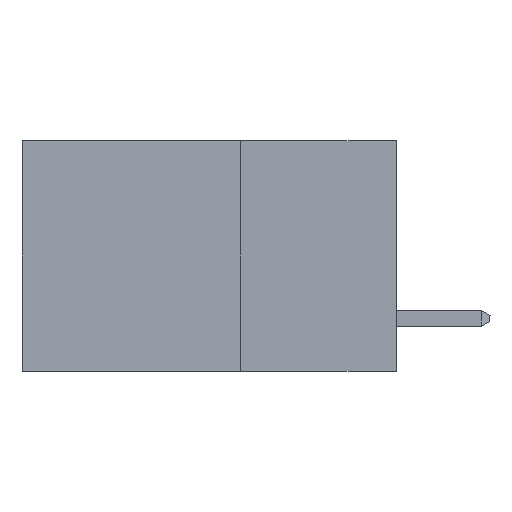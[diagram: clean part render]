
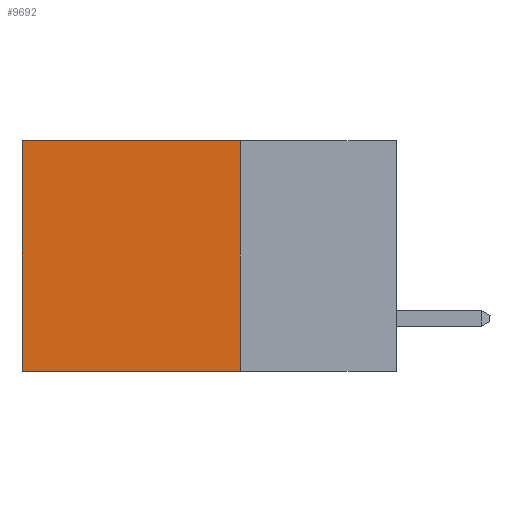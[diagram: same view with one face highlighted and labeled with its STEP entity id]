
A CAD part, left-side view. The second image highlights one B-rep face of the part: STEP entity #9692.
In plain terms, the highlighted planar face has unit normal (-1, 0, 0).
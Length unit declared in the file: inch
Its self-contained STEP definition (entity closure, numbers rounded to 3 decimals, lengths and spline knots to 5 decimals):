
#252 = VECTOR ( 'NONE', #7902, 39.37008 ) ;
#567 = EDGE_LOOP ( 'NONE', ( #10667, #6656, #911, #1092 ) ) ;
#683 = CARTESIAN_POINT ( 'NONE',  ( 0.298, 0.6, -0.37 ) ) ;
#911 = ORIENTED_EDGE ( 'NONE', *, *, #4705, .F. ) ;
#1075 = VERTEX_POINT ( 'NONE', #6024 ) ;
#1092 = ORIENTED_EDGE ( 'NONE', *, *, #1733, .T. ) ;
#1318 = CARTESIAN_POINT ( 'NONE',  ( 0.298, 0.25, -0.37 ) ) ;
#1333 = CARTESIAN_POINT ( 'NONE',  ( 0.298, 0.25, 0. ) ) ;
#1408 = LINE ( 'NONE', #6724, #8051 ) ;
#1498 = FACE_OUTER_BOUND ( 'NONE', #567, .T. ) ;
#1511 = VERTEX_POINT ( 'NONE', #3135 ) ;
#1540 = CARTESIAN_POINT ( 'NONE',  ( 0.298, 0.25, 0. ) ) ;
#1733 = EDGE_CURVE ( 'NONE', #1075, #1511, #1964, .T. ) ;
#1777 = DIRECTION ( 'NONE',  ( 0., 0., -1. ) ) ;
#1964 = LINE ( 'NONE', #1540, #252 ) ;
#2083 = DIRECTION ( 'NONE',  ( 0., 1., 0. ) ) ;
#2366 = DIRECTION ( 'NONE',  ( 0., 0., -1. ) ) ;
#2425 = VERTEX_POINT ( 'NONE', #683 ) ;
#3135 = CARTESIAN_POINT ( 'NONE',  ( 0.298, 0.6, 0. ) ) ;
#3507 = AXIS2_PLACEMENT_3D ( 'NONE', #7560, #3572, #1777 ) ;
#3572 = DIRECTION ( 'NONE',  ( 1., 0., 0. ) ) ;
#3869 = VECTOR ( 'NONE', #8959, 39.37008 ) ;
#4705 = EDGE_CURVE ( 'NONE', #1075, #8043, #5598, .T. ) ;
#5598 = LINE ( 'NONE', #1333, #3869 ) ;
#6024 = CARTESIAN_POINT ( 'NONE',  ( 0.298, 0.25, 0. ) ) ;
#6656 = ORIENTED_EDGE ( 'NONE', *, *, #7917, .F. ) ;
#6692 = PLANE ( 'NONE',  #3507 ) ;
#6704 = EDGE_CURVE ( 'NONE', #1511, #2425, #10467, .T. ) ;
#6724 = CARTESIAN_POINT ( 'NONE',  ( 0.298, 0.25, -0.37 ) ) ;
#7560 = CARTESIAN_POINT ( 'NONE',  ( 0.298, 0.25, 0. ) ) ;
#7902 = DIRECTION ( 'NONE',  ( 0., 1., 0. ) ) ;
#7917 = EDGE_CURVE ( 'NONE', #8043, #2425, #1408, .T. ) ;
#8043 = VERTEX_POINT ( 'NONE', #1318 ) ;
#8051 = VECTOR ( 'NONE', #2083, 39.37008 ) ;
#8959 = DIRECTION ( 'NONE',  ( 0., 0., -1. ) ) ;
#9692 = ADVANCED_FACE ( 'NONE', ( #1498 ), #6692, .F. ) ;
#10467 = LINE ( 'NONE', #10822, #10602 ) ;
#10602 = VECTOR ( 'NONE', #2366, 39.37008 ) ;
#10667 = ORIENTED_EDGE ( 'NONE', *, *, #6704, .T. ) ;
#10822 = CARTESIAN_POINT ( 'NONE',  ( 0.298, 0.6, 0. ) ) ;
